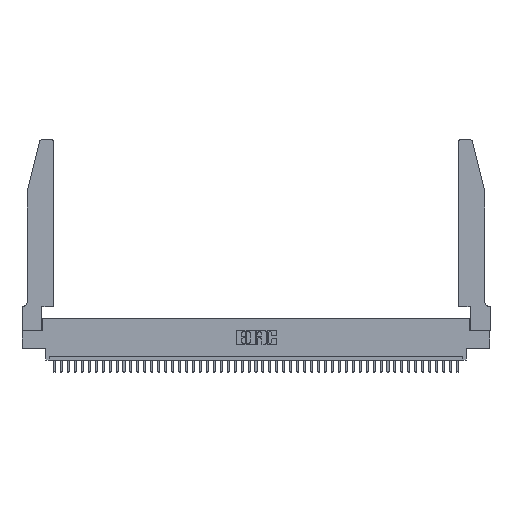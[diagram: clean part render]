
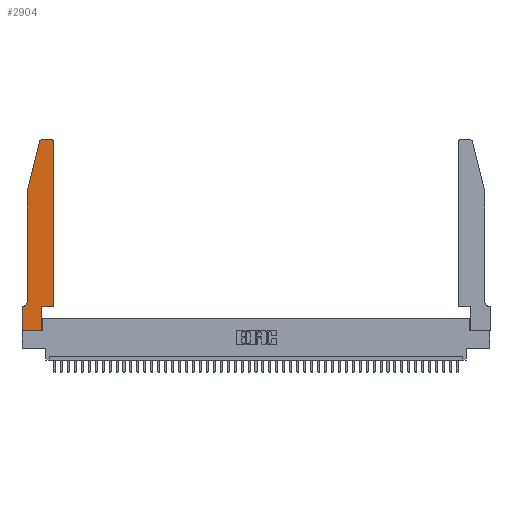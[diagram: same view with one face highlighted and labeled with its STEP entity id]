
A CAD part, top view. The second image highlights one B-rep face of the part: STEP entity #2904.
In plain terms, the highlighted planar face has unit normal (0, 0, 1).
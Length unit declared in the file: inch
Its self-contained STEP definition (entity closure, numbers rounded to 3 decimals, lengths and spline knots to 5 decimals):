
#801 = ORIENTED_EDGE ( 'NONE', *, *, #43281, .T. ) ;
#872 = ORIENTED_EDGE ( 'NONE', *, *, #40371, .T. ) ;
#1078 = ORIENTED_EDGE ( 'NONE', *, *, #15532, .T. ) ;
#1465 = VECTOR ( 'NONE', #5828, 39.37008 ) ;
#2159 = CARTESIAN_POINT ( 'NONE',  ( 0.0755, 0.35, 0.37 ) ) ;
#2766 = VECTOR ( 'NONE', #30406, 39.37008 ) ;
#2833 = ORIENTED_EDGE ( 'NONE', *, *, #19008, .T. ) ;
#2904 = ADVANCED_FACE ( 'NONE', ( #13648 ), #12521, .T. ) ;
#2995 = DIRECTION ( 'NONE',  ( 1., 0., 0. ) ) ;
#3316 = LINE ( 'NONE', #9251, #7287 ) ;
#3883 = ORIENTED_EDGE ( 'NONE', *, *, #27325, .T. ) ;
#4069 = VERTEX_POINT ( 'NONE', #25686 ) ;
#5368 = EDGE_LOOP ( 'NONE', ( #24305, #18669, #1078, #872, #3883, #38433, #15680, #2833, #16207, #34538, #801, #6379 ) ) ;
#5536 = CARTESIAN_POINT ( 'NONE',  ( 0., 0.35, 0.37 ) ) ;
#5828 = DIRECTION ( 'NONE',  ( -1., 0., 0. ) ) ;
#6379 = ORIENTED_EDGE ( 'NONE', *, *, #20642, .T. ) ;
#6914 = AXIS2_PLACEMENT_3D ( 'NONE', #44301, #33656, #22793 ) ;
#7287 = VECTOR ( 'NONE', #31601, 39.37008 ) ;
#7423 = EDGE_CURVE ( 'NONE', #38282, #25939, #10056, .T. ) ;
#8585 = DIRECTION ( 'NONE',  ( 0., 0., -1. ) ) ;
#9251 = CARTESIAN_POINT ( 'NONE',  ( 0.2605, 2.75, 0.37 ) ) ;
#10056 = CIRCLE ( 'NONE', #6914, 0.03 ) ;
#11081 = VERTEX_POINT ( 'NONE', #40519 ) ;
#11809 = CARTESIAN_POINT ( 'NONE',  ( 0.284, 2.75, 0.37 ) ) ;
#12237 = CARTESIAN_POINT ( 'NONE',  ( 0.0055, 0.42, 0.37 ) ) ;
#12371 = VERTEX_POINT ( 'NONE', #15403 ) ;
#12521 = PLANE ( 'NONE',  #39925 ) ;
#12630 = AXIS2_PLACEMENT_3D ( 'NONE', #46546, #35706, #2995 ) ;
#13648 = FACE_OUTER_BOUND ( 'NONE', #5368, .T. ) ;
#14408 = CARTESIAN_POINT ( 'NONE',  ( 0.2865, 0.35, 0.37 ) ) ;
#15403 = CARTESIAN_POINT ( 'NONE',  ( 0.4505, 0.35, 0.37 ) ) ;
#15532 = EDGE_CURVE ( 'NONE', #25939, #4069, #21571, .T. ) ;
#15570 = DIRECTION ( 'NONE',  ( 0., -1., 0. ) ) ;
#15680 = ORIENTED_EDGE ( 'NONE', *, *, #36507, .T. ) ;
#15823 = VECTOR ( 'NONE', #16068, 39.37008 ) ;
#16068 = DIRECTION ( 'NONE',  ( 0., -1., 0. ) ) ;
#16153 = DIRECTION ( 'NONE',  ( 0., 0., 1. ) ) ;
#16207 = ORIENTED_EDGE ( 'NONE', *, *, #23663, .T. ) ;
#16377 = CARTESIAN_POINT ( 'NONE',  ( 0.0755, 2., 0.37 ) ) ;
#18141 = CARTESIAN_POINT ( 'NONE',  ( 0.25487, 2.72718, 0.37 ) ) ;
#18166 = VERTEX_POINT ( 'NONE', #14408 ) ;
#18669 = ORIENTED_EDGE ( 'NONE', *, *, #7423, .T. ) ;
#19008 = EDGE_CURVE ( 'NONE', #33760, #31835, #30728, .T. ) ;
#19827 = VERTEX_POINT ( 'NONE', #37360 ) ;
#20498 = EDGE_CURVE ( 'NONE', #18166, #12371, #30864, .T. ) ;
#20642 = EDGE_CURVE ( 'NONE', #31972, #19827, #31966, .T. ) ;
#21033 = VECTOR ( 'NONE', #39754, 39.37008 ) ;
#21172 = VECTOR ( 'NONE', #30798, 39.37008 ) ;
#21527 = CIRCLE ( 'NONE', #44141, 0.07 ) ;
#21571 = LINE ( 'NONE', #43484, #25002 ) ;
#21650 = DIRECTION ( 'NONE',  ( -0.239, -0.971, 0. ) ) ;
#22719 = VERTEX_POINT ( 'NONE', #28870 ) ;
#22793 = DIRECTION ( 'NONE',  ( 1., 0., 0. ) ) ;
#22980 = CARTESIAN_POINT ( 'NONE',  ( 0.4505, 0.35, 0.37 ) ) ;
#23124 = DIRECTION ( 'NONE',  ( 1., 0., 0. ) ) ;
#23663 = EDGE_CURVE ( 'NONE', #31835, #18166, #40264, .T. ) ;
#24305 = ORIENTED_EDGE ( 'NONE', *, *, #28168, .T. ) ;
#25002 = VECTOR ( 'NONE', #21650, 39.37008 ) ;
#25686 = CARTESIAN_POINT ( 'NONE',  ( 0.0755, 2., 0.37 ) ) ;
#25939 = VERTEX_POINT ( 'NONE', #18141 ) ;
#25941 = LINE ( 'NONE', #16377, #15823 ) ;
#26581 = CARTESIAN_POINT ( 'NONE',  ( 0.2865, 0.35, 0.37 ) ) ;
#27325 = EDGE_CURVE ( 'NONE', #22719, #11081, #21527, .T. ) ;
#28168 = EDGE_CURVE ( 'NONE', #19827, #38282, #3316, .T. ) ;
#28870 = CARTESIAN_POINT ( 'NONE',  ( 0.0755, 0.42, 0.37 ) ) ;
#29385 = CARTESIAN_POINT ( 'NONE',  ( 0., 0., 0.37 ) ) ;
#29685 = CARTESIAN_POINT ( 'NONE',  ( 0., 0., 0.37 ) ) ;
#30406 = DIRECTION ( 'NONE',  ( 0., 1., 0. ) ) ;
#30728 = LINE ( 'NONE', #29385, #21033 ) ;
#30798 = DIRECTION ( 'NONE',  ( 1., 0., 0. ) ) ;
#30864 = LINE ( 'NONE', #30954, #21172 ) ;
#30954 = CARTESIAN_POINT ( 'NONE',  ( 0.4505, 0.35, 0.37 ) ) ;
#31601 = DIRECTION ( 'NONE',  ( -1., 0., 0. ) ) ;
#31835 = VERTEX_POINT ( 'NONE', #42906 ) ;
#31966 = CIRCLE ( 'NONE', #12630, 0.03 ) ;
#31972 = VERTEX_POINT ( 'NONE', #33017 ) ;
#32570 = VECTOR ( 'NONE', #44657, 39.37008 ) ;
#33017 = CARTESIAN_POINT ( 'NONE',  ( 0.4505, 2.72, 0.37 ) ) ;
#33656 = DIRECTION ( 'NONE',  ( 0., 0., 1. ) ) ;
#33760 = VERTEX_POINT ( 'NONE', #38898 ) ;
#34436 = LINE ( 'NONE', #2159, #1465 ) ;
#34538 = ORIENTED_EDGE ( 'NONE', *, *, #20498, .T. ) ;
#35706 = DIRECTION ( 'NONE',  ( 0., 0., 1. ) ) ;
#36507 = EDGE_CURVE ( 'NONE', #46017, #33760, #46224, .T. ) ;
#36534 = VECTOR ( 'NONE', #15570, 39.37008 ) ;
#37314 = DIRECTION ( 'NONE',  ( -1., 0., 0. ) ) ;
#37360 = CARTESIAN_POINT ( 'NONE',  ( 0.4205, 2.75, 0.37 ) ) ;
#38282 = VERTEX_POINT ( 'NONE', #11809 ) ;
#38433 = ORIENTED_EDGE ( 'NONE', *, *, #41789, .T. ) ;
#38898 = CARTESIAN_POINT ( 'NONE',  ( 0., 0., 0.37 ) ) ;
#39754 = DIRECTION ( 'NONE',  ( 1., 0., 0. ) ) ;
#39925 = AXIS2_PLACEMENT_3D ( 'NONE', #5536, #16153, #23124 ) ;
#40264 = LINE ( 'NONE', #26581, #2766 ) ;
#40371 = EDGE_CURVE ( 'NONE', #4069, #22719, #25941, .T. ) ;
#40519 = CARTESIAN_POINT ( 'NONE',  ( 0.0055, 0.35, 0.37 ) ) ;
#41789 = EDGE_CURVE ( 'NONE', #11081, #46017, #34436, .T. ) ;
#42906 = CARTESIAN_POINT ( 'NONE',  ( 0.2865, 0., 0.37 ) ) ;
#43281 = EDGE_CURVE ( 'NONE', #12371, #31972, #43383, .T. ) ;
#43383 = LINE ( 'NONE', #22980, #32570 ) ;
#43484 = CARTESIAN_POINT ( 'NONE',  ( 0.0755, 2., 0.37 ) ) ;
#44141 = AXIS2_PLACEMENT_3D ( 'NONE', #12237, #8585, #37314 ) ;
#44301 = CARTESIAN_POINT ( 'NONE',  ( 0.284, 2.72, 0.37 ) ) ;
#44657 = DIRECTION ( 'NONE',  ( 0., 1., 0. ) ) ;
#46017 = VERTEX_POINT ( 'NONE', #46477 ) ;
#46224 = LINE ( 'NONE', #29685, #36534 ) ;
#46477 = CARTESIAN_POINT ( 'NONE',  ( 0., 0.35, 0.37 ) ) ;
#46546 = CARTESIAN_POINT ( 'NONE',  ( 0.4205, 2.72, 0.37 ) ) ;
